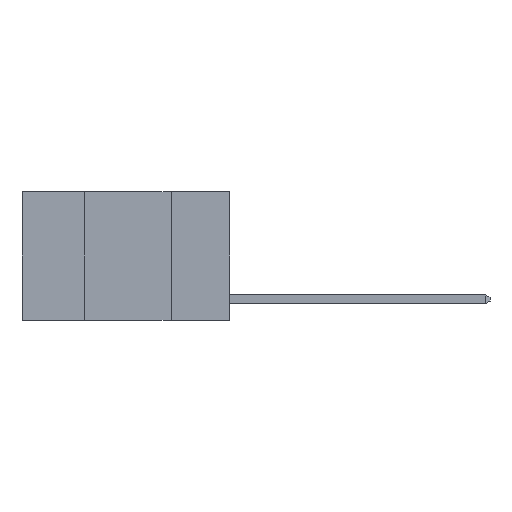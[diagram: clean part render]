
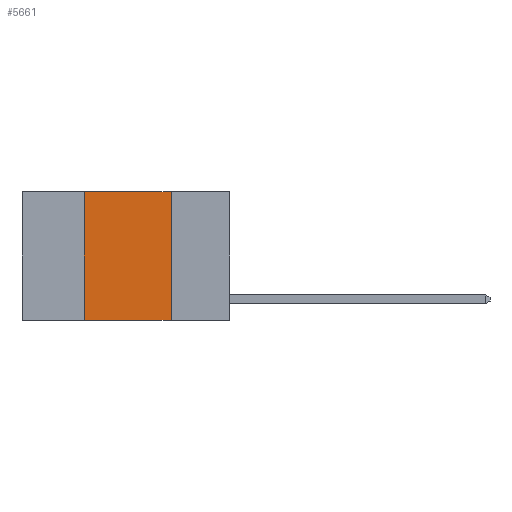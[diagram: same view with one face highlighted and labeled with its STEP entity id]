
A CAD part, left-side view. The second image highlights one B-rep face of the part: STEP entity #5661.
In plain terms, the highlighted planar face has unit normal (-1, 0, 0).
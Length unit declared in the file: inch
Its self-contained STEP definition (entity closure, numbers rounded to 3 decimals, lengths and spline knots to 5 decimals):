
#75 = CARTESIAN_POINT ( 'NONE',  ( 0., 0.6, -0.37 ) ) ;
#136 = DIRECTION ( 'NONE',  ( 1., 0., 0. ) ) ;
#433 = VERTEX_POINT ( 'NONE', #6992 ) ;
#670 = VECTOR ( 'NONE', #5091, 39.37008 ) ;
#980 = FACE_OUTER_BOUND ( 'NONE', #7556, .T. ) ;
#1081 = EDGE_CURVE ( 'NONE', #1426, #3586, #9879, .T. ) ;
#1121 = CARTESIAN_POINT ( 'NONE',  ( 0., 0.17, 0. ) ) ;
#1426 = VERTEX_POINT ( 'NONE', #1612 ) ;
#1612 = CARTESIAN_POINT ( 'NONE',  ( 0., 0.17, 0. ) ) ;
#2049 = VERTEX_POINT ( 'NONE', #11170 ) ;
#2545 = ORIENTED_EDGE ( 'NONE', *, *, #6877, .T. ) ;
#2582 = VECTOR ( 'NONE', #8117, 39.37008 ) ;
#3584 = DIRECTION ( 'NONE',  ( 0., -1., 0. ) ) ;
#3586 = VERTEX_POINT ( 'NONE', #5365 ) ;
#3761 = LINE ( 'NONE', #75, #10226 ) ;
#4409 = LINE ( 'NONE', #10025, #9107 ) ;
#4742 = DIRECTION ( 'NONE',  ( 0., -1., 0. ) ) ;
#5091 = DIRECTION ( 'NONE',  ( 0., 0., 1. ) ) ;
#5365 = CARTESIAN_POINT ( 'NONE',  ( 0., 0.17, -0.37 ) ) ;
#5375 = CARTESIAN_POINT ( 'NONE',  ( 0., 0.6, 0. ) ) ;
#5661 = ADVANCED_FACE ( 'NONE', ( #980 ), #9777, .F. ) ;
#6247 = ORIENTED_EDGE ( 'NONE', *, *, #8275, .F. ) ;
#6256 = DIRECTION ( 'NONE',  ( 0., 0., -1. ) ) ;
#6877 = EDGE_CURVE ( 'NONE', #433, #3586, #3761, .T. ) ;
#6992 = CARTESIAN_POINT ( 'NONE',  ( 0., 0.42, -0.37 ) ) ;
#7556 = EDGE_LOOP ( 'NONE', ( #11174, #6247, #9342, #2545 ) ) ;
#8117 = DIRECTION ( 'NONE',  ( 0., 0., -1. ) ) ;
#8275 = EDGE_CURVE ( 'NONE', #2049, #1426, #4409, .T. ) ;
#9107 = VECTOR ( 'NONE', #4742, 39.37008 ) ;
#9342 = ORIENTED_EDGE ( 'NONE', *, *, #10951, .F. ) ;
#9777 = PLANE ( 'NONE',  #10676 ) ;
#9879 = LINE ( 'NONE', #1121, #2582 ) ;
#10025 = CARTESIAN_POINT ( 'NONE',  ( 0., 0.6, 0. ) ) ;
#10226 = VECTOR ( 'NONE', #3584, 39.37008 ) ;
#10277 = LINE ( 'NONE', #10363, #670 ) ;
#10363 = CARTESIAN_POINT ( 'NONE',  ( 0., 0.42, 0. ) ) ;
#10676 = AXIS2_PLACEMENT_3D ( 'NONE', #5375, #136, #6256 ) ;
#10951 = EDGE_CURVE ( 'NONE', #433, #2049, #10277, .T. ) ;
#11170 = CARTESIAN_POINT ( 'NONE',  ( 0., 0.42, 0. ) ) ;
#11174 = ORIENTED_EDGE ( 'NONE', *, *, #1081, .F. ) ;
